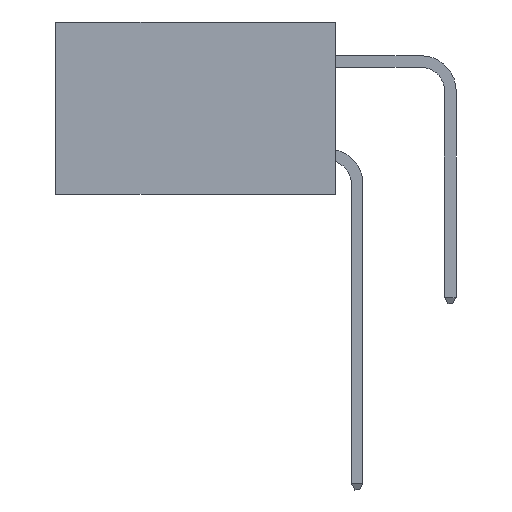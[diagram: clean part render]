
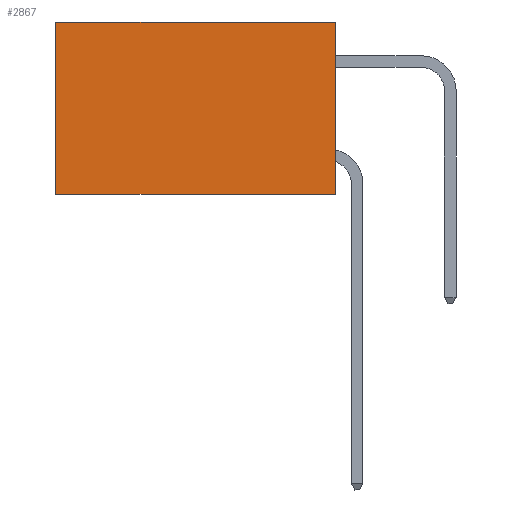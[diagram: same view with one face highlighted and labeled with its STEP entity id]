
A CAD part, left-side view. The second image highlights one B-rep face of the part: STEP entity #2867.
In plain terms, the highlighted planar face has unit normal (-1, 0, 0).
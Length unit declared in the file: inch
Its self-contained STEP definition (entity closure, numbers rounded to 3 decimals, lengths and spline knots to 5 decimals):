
#976 = CARTESIAN_POINT ( 'NONE',  ( 0.2875, 0., 0. ) ) ;
#2619 = ORIENTED_EDGE ( 'NONE', *, *, #4099, .F. ) ;
#2768 = VECTOR ( 'NONE', #22272, 39.37008 ) ;
#2867 = ADVANCED_FACE ( 'NONE', ( #4473 ), #9022, .F. ) ;
#2884 = VERTEX_POINT ( 'NONE', #23638 ) ;
#4099 = EDGE_CURVE ( 'NONE', #21313, #5288, #29951, .T. ) ;
#4473 = FACE_OUTER_BOUND ( 'NONE', #28256, .T. ) ;
#5288 = VERTEX_POINT ( 'NONE', #22092 ) ;
#6084 = EDGE_CURVE ( 'NONE', #2884, #21247, #15145, .T. ) ;
#6386 = ORIENTED_EDGE ( 'NONE', *, *, #6084, .T. ) ;
#7131 = CARTESIAN_POINT ( 'NONE',  ( 0.2875, 0.6, 0. ) ) ;
#8222 = CARTESIAN_POINT ( 'NONE',  ( 0.2875, 0., -0.37 ) ) ;
#8501 = VECTOR ( 'NONE', #25651, 39.37008 ) ;
#9022 = PLANE ( 'NONE',  #27146 ) ;
#11804 = ORIENTED_EDGE ( 'NONE', *, *, #16488, .T. ) ;
#12021 = CARTESIAN_POINT ( 'NONE',  ( 0.2875, 0., -0.37 ) ) ;
#12188 = ORIENTED_EDGE ( 'NONE', *, *, #19280, .F. ) ;
#12262 = DIRECTION ( 'NONE',  ( 0., 0., -1. ) ) ;
#12535 = LINE ( 'NONE', #14516, #28708 ) ;
#13447 = VECTOR ( 'NONE', #23278, 39.37008 ) ;
#14516 = CARTESIAN_POINT ( 'NONE',  ( 0.2875, 0., 0. ) ) ;
#15145 = LINE ( 'NONE', #976, #2768 ) ;
#16166 = DIRECTION ( 'NONE',  ( 1., 0., 0. ) ) ;
#16488 = EDGE_CURVE ( 'NONE', #21247, #5288, #23590, .T. ) ;
#19280 = EDGE_CURVE ( 'NONE', #2884, #21313, #12535, .T. ) ;
#20746 = CARTESIAN_POINT ( 'NONE',  ( 0.2875, 0.6, 0. ) ) ;
#21247 = VERTEX_POINT ( 'NONE', #7131 ) ;
#21313 = VERTEX_POINT ( 'NONE', #12021 ) ;
#22092 = CARTESIAN_POINT ( 'NONE',  ( 0.2875, 0.6, -0.37 ) ) ;
#22272 = DIRECTION ( 'NONE',  ( 0., 1., 0. ) ) ;
#23278 = DIRECTION ( 'NONE',  ( 0., 0., -1. ) ) ;
#23332 = DIRECTION ( 'NONE',  ( 0., 0., -1. ) ) ;
#23590 = LINE ( 'NONE', #20746, #13447 ) ;
#23638 = CARTESIAN_POINT ( 'NONE',  ( 0.2875, 0., 0. ) ) ;
#25651 = DIRECTION ( 'NONE',  ( 0., 1., 0. ) ) ;
#27146 = AXIS2_PLACEMENT_3D ( 'NONE', #30791, #16166, #23332 ) ;
#28256 = EDGE_LOOP ( 'NONE', ( #11804, #2619, #12188, #6386 ) ) ;
#28708 = VECTOR ( 'NONE', #12262, 39.37008 ) ;
#29951 = LINE ( 'NONE', #8222, #8501 ) ;
#30791 = CARTESIAN_POINT ( 'NONE',  ( 0.2875, 0., 0. ) ) ;
